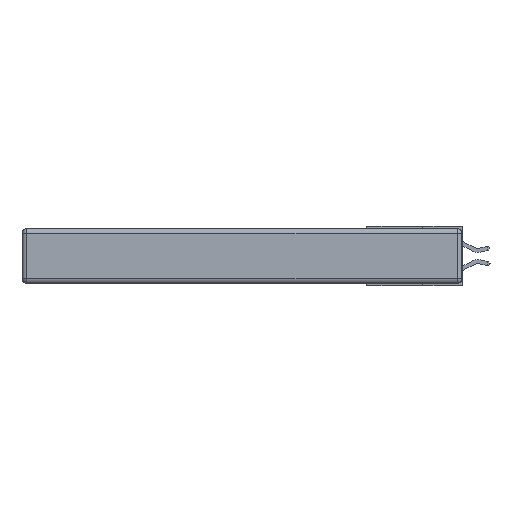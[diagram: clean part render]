
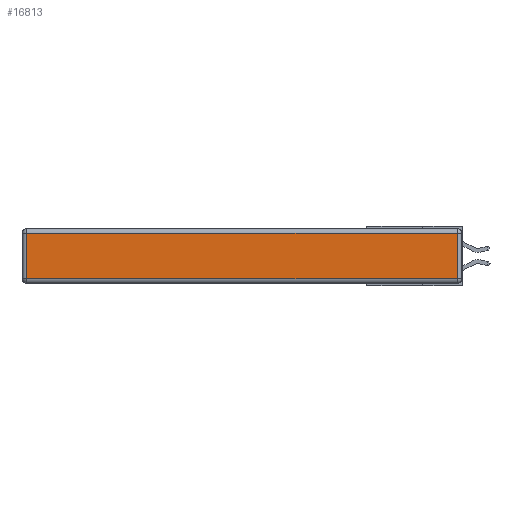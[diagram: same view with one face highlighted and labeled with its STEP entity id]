
A CAD part, left-side view. The second image highlights one B-rep face of the part: STEP entity #16813.
In plain terms, the highlighted planar face has unit normal (-1, 0, 0).
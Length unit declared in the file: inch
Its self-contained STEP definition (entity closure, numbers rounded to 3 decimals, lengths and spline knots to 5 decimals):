
#1532 = CARTESIAN_POINT ( 'NONE',  ( 0., 2.72, -0.343 ) ) ;
#1853 = CARTESIAN_POINT ( 'NONE',  ( 0., 2.72, -0.03 ) ) ;
#2171 = CARTESIAN_POINT ( 'NONE',  ( 0., 0.03, -0.343 ) ) ;
#3509 = DIRECTION ( 'NONE',  ( 0., 1., 0. ) ) ;
#3786 = VERTEX_POINT ( 'NONE', #7874 ) ;
#5177 = ORIENTED_EDGE ( 'NONE', *, *, #5504, .T. ) ;
#5504 = EDGE_CURVE ( 'NONE', #13629, #12865, #7472, .T. ) ;
#5631 = CARTESIAN_POINT ( 'NONE',  ( 0., 0., -0.343 ) ) ;
#5881 = CARTESIAN_POINT ( 'NONE',  ( 0., 0.03, -0.03 ) ) ;
#6481 = VECTOR ( 'NONE', #15975, 39.37008 ) ;
#6663 = LINE ( 'NONE', #2171, #16913 ) ;
#7472 = LINE ( 'NONE', #1532, #6481 ) ;
#7874 = CARTESIAN_POINT ( 'NONE',  ( 0., 0.03, -0.313 ) ) ;
#8517 = FACE_OUTER_BOUND ( 'NONE', #13632, .T. ) ;
#8549 = LINE ( 'NONE', #9978, #10303 ) ;
#8564 = DIRECTION ( 'NONE',  ( 0., -1., 0. ) ) ;
#8688 = EDGE_CURVE ( 'NONE', #12865, #3786, #9101, .T. ) ;
#8901 = PLANE ( 'NONE',  #14644 ) ;
#9101 = LINE ( 'NONE', #19784, #10834 ) ;
#9978 = CARTESIAN_POINT ( 'NONE',  ( 0., 2.75, -0.03 ) ) ;
#10089 = EDGE_CURVE ( 'NONE', #13070, #13629, #8549, .T. ) ;
#10303 = VECTOR ( 'NONE', #3509, 39.37008 ) ;
#10834 = VECTOR ( 'NONE', #8564, 39.37008 ) ;
#11628 = EDGE_CURVE ( 'NONE', #3786, #13070, #6663, .T. ) ;
#12362 = DIRECTION ( 'NONE',  ( 0., 0., 1. ) ) ;
#12865 = VERTEX_POINT ( 'NONE', #19029 ) ;
#13070 = VERTEX_POINT ( 'NONE', #5881 ) ;
#13102 = DIRECTION ( 'NONE',  ( 0., 0., 1. ) ) ;
#13252 = DIRECTION ( 'NONE',  ( -1., 0., 0. ) ) ;
#13629 = VERTEX_POINT ( 'NONE', #1853 ) ;
#13632 = EDGE_LOOP ( 'NONE', ( #15526, #19460, #15564, #5177 ) ) ;
#14644 = AXIS2_PLACEMENT_3D ( 'NONE', #5631, #13252, #13102 ) ;
#15526 = ORIENTED_EDGE ( 'NONE', *, *, #8688, .T. ) ;
#15564 = ORIENTED_EDGE ( 'NONE', *, *, #10089, .T. ) ;
#15975 = DIRECTION ( 'NONE',  ( 0., 0., -1. ) ) ;
#16813 = ADVANCED_FACE ( 'NONE', ( #8517 ), #8901, .T. ) ;
#16913 = VECTOR ( 'NONE', #12362, 39.37008 ) ;
#19029 = CARTESIAN_POINT ( 'NONE',  ( 0., 2.72, -0.313 ) ) ;
#19460 = ORIENTED_EDGE ( 'NONE', *, *, #11628, .T. ) ;
#19784 = CARTESIAN_POINT ( 'NONE',  ( 0., 0., -0.313 ) ) ;
